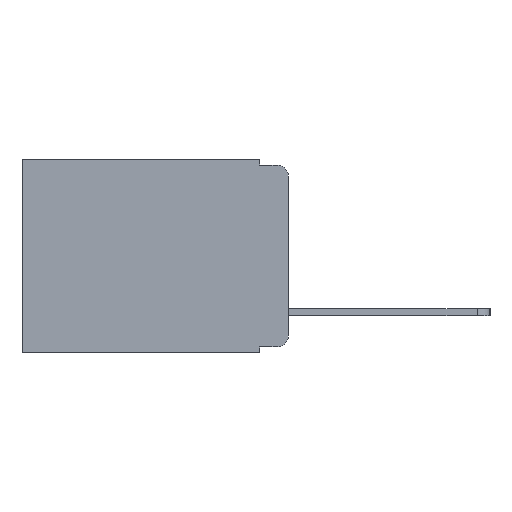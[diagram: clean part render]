
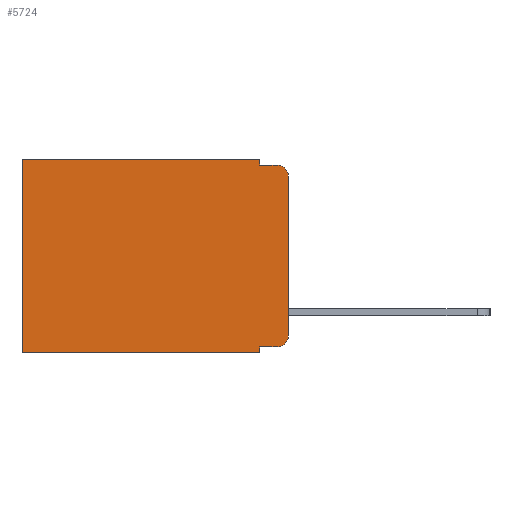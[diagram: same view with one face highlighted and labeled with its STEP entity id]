
A CAD part, left-side view. The second image highlights one B-rep face of the part: STEP entity #5724.
In plain terms, the highlighted planar face has unit normal (-1, 0, 0).
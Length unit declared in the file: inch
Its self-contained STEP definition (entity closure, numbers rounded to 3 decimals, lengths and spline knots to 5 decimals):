
#82 = ORIENTED_EDGE ( 'NONE', *, *, #8377, .T. ) ;
#190 = ORIENTED_EDGE ( 'NONE', *, *, #8359, .F. ) ;
#415 = VERTEX_POINT ( 'NONE', #7577 ) ;
#423 = DIRECTION ( 'NONE',  ( 0., 0., -1. ) ) ;
#771 = VERTEX_POINT ( 'NONE', #3663 ) ;
#979 = ORIENTED_EDGE ( 'NONE', *, *, #1077, .F. ) ;
#1007 = ORIENTED_EDGE ( 'NONE', *, *, #5299, .T. ) ;
#1014 = CARTESIAN_POINT ( 'NONE',  ( 0.298, 0.02, -0.333 ) ) ;
#1077 = EDGE_CURVE ( 'NONE', #7896, #415, #3103, .T. ) ;
#1097 = CARTESIAN_POINT ( 'NONE',  ( 0.298, 0.473, 0. ) ) ;
#1427 = DIRECTION ( 'NONE',  ( 0., 1., 0. ) ) ;
#1825 = DIRECTION ( 'NONE',  ( 0., 0., -1. ) ) ;
#1996 = AXIS2_PLACEMENT_3D ( 'NONE', #7749, #2666, #8629 ) ;
#2127 = VERTEX_POINT ( 'NONE', #1014 ) ;
#2159 = CARTESIAN_POINT ( 'NONE',  ( 0.298, 0.051, -0.01 ) ) ;
#2296 = ORIENTED_EDGE ( 'NONE', *, *, #4402, .T. ) ;
#2313 = DIRECTION ( 'NONE',  ( 0., -1., 0. ) ) ;
#2457 = ORIENTED_EDGE ( 'NONE', *, *, #10166, .T. ) ;
#2502 = VERTEX_POINT ( 'NONE', #7843 ) ;
#2626 = DIRECTION ( 'NONE',  ( 0., 1., 0. ) ) ;
#2666 = DIRECTION ( 'NONE',  ( -1., 0., 0. ) ) ;
#2675 = CARTESIAN_POINT ( 'NONE',  ( 0.298, 0., -0.03 ) ) ;
#2766 = CARTESIAN_POINT ( 'NONE',  ( 0.298, 0.473, 0. ) ) ;
#2996 = LINE ( 'NONE', #6243, #9553 ) ;
#3103 = LINE ( 'NONE', #9639, #4850 ) ;
#3248 = VECTOR ( 'NONE', #6937, 39.37008 ) ;
#3354 = ORIENTED_EDGE ( 'NONE', *, *, #10313, .F. ) ;
#3479 = FACE_OUTER_BOUND ( 'NONE', #9090, .T. ) ;
#3663 = CARTESIAN_POINT ( 'NONE',  ( 0.298, 0.02, -0.01 ) ) ;
#4377 = EDGE_CURVE ( 'NONE', #10200, #8813, #5758, .T. ) ;
#4380 = VERTEX_POINT ( 'NONE', #6906 ) ;
#4402 = EDGE_CURVE ( 'NONE', #2502, #6984, #2996, .T. ) ;
#4721 = CIRCLE ( 'NONE', #7910, 0.02 ) ;
#4850 = VECTOR ( 'NONE', #423, 39.37008 ) ;
#4919 = DIRECTION ( 'NONE',  ( -1., 0., 0. ) ) ;
#5036 = PLANE ( 'NONE',  #10407 ) ;
#5223 = VECTOR ( 'NONE', #8482, 39.37008 ) ;
#5299 = EDGE_CURVE ( 'NONE', #6984, #4380, #9792, .T. ) ;
#5338 = CARTESIAN_POINT ( 'NONE',  ( 0.298, 0.051, 0. ) ) ;
#5356 = LINE ( 'NONE', #6242, #7105 ) ;
#5380 = DIRECTION ( 'NONE',  ( 0., 0., -1. ) ) ;
#5655 = CIRCLE ( 'NONE', #1996, 0.02 ) ;
#5724 = ADVANCED_FACE ( 'NONE', ( #3479 ), #5036, .F. ) ;
#5758 = LINE ( 'NONE', #5338, #3248 ) ;
#6135 = ORIENTED_EDGE ( 'NONE', *, *, #4377, .F. ) ;
#6159 = ORIENTED_EDGE ( 'NONE', *, *, #10584, .T. ) ;
#6242 = CARTESIAN_POINT ( 'NONE',  ( 0.298, 0.051, 0. ) ) ;
#6243 = CARTESIAN_POINT ( 'NONE',  ( 0.298, 0., 0. ) ) ;
#6434 = VECTOR ( 'NONE', #9492, 39.37008 ) ;
#6581 = CARTESIAN_POINT ( 'NONE',  ( 0.298, 0.051, -0.343 ) ) ;
#6906 = CARTESIAN_POINT ( 'NONE',  ( 0.298, 0.473, -0.343 ) ) ;
#6937 = DIRECTION ( 'NONE',  ( 0., 0., -1. ) ) ;
#6984 = VERTEX_POINT ( 'NONE', #2766 ) ;
#7105 = VECTOR ( 'NONE', #5380, 39.37008 ) ;
#7117 = VECTOR ( 'NONE', #2313, 39.37008 ) ;
#7375 = LINE ( 'NONE', #8262, #7117 ) ;
#7577 = CARTESIAN_POINT ( 'NONE',  ( 0.298, 0., -0.313 ) ) ;
#7719 = CARTESIAN_POINT ( 'NONE',  ( 0.298, 0., -0.343 ) ) ;
#7749 = CARTESIAN_POINT ( 'NONE',  ( 0.298, 0.02, -0.03 ) ) ;
#7833 = DIRECTION ( 'NONE',  ( 1., 0., 0. ) ) ;
#7843 = CARTESIAN_POINT ( 'NONE',  ( 0.298, 0.051, 0. ) ) ;
#7896 = VERTEX_POINT ( 'NONE', #2675 ) ;
#7910 = AXIS2_PLACEMENT_3D ( 'NONE', #10032, #4919, #10851 ) ;
#8150 = ORIENTED_EDGE ( 'NONE', *, *, #9909, .F. ) ;
#8207 = VECTOR ( 'NONE', #2626, 39.37008 ) ;
#8262 = CARTESIAN_POINT ( 'NONE',  ( 0.298, 0.051, -0.01 ) ) ;
#8359 = EDGE_CURVE ( 'NONE', #8813, #4380, #10484, .T. ) ;
#8377 = EDGE_CURVE ( 'NONE', #7896, #771, #5655, .T. ) ;
#8482 = DIRECTION ( 'NONE',  ( 0., 0., -1. ) ) ;
#8614 = CARTESIAN_POINT ( 'NONE',  ( 0.298, 0.051, -0.333 ) ) ;
#8629 = DIRECTION ( 'NONE',  ( 0., 0., -1. ) ) ;
#8813 = VERTEX_POINT ( 'NONE', #6581 ) ;
#9090 = EDGE_LOOP ( 'NONE', ( #979, #82, #8150, #3354, #2296, #1007, #190, #6135, #2457, #6159 ) ) ;
#9418 = CARTESIAN_POINT ( 'NONE',  ( 0.298, 0., 0. ) ) ;
#9492 = DIRECTION ( 'NONE',  ( 0., -1., 0. ) ) ;
#9522 = CARTESIAN_POINT ( 'NONE',  ( 0.298, 0.051, -0.333 ) ) ;
#9553 = VECTOR ( 'NONE', #1427, 39.37008 ) ;
#9639 = CARTESIAN_POINT ( 'NONE',  ( 0.298, 0., 0. ) ) ;
#9792 = LINE ( 'NONE', #1097, #5223 ) ;
#9909 = EDGE_CURVE ( 'NONE', #10448, #771, #7375, .T. ) ;
#10032 = CARTESIAN_POINT ( 'NONE',  ( 0.298, 0.02, -0.313 ) ) ;
#10166 = EDGE_CURVE ( 'NONE', #10200, #2127, #10955, .T. ) ;
#10200 = VERTEX_POINT ( 'NONE', #9522 ) ;
#10313 = EDGE_CURVE ( 'NONE', #2502, #10448, #5356, .T. ) ;
#10407 = AXIS2_PLACEMENT_3D ( 'NONE', #9418, #7833, #1825 ) ;
#10448 = VERTEX_POINT ( 'NONE', #2159 ) ;
#10484 = LINE ( 'NONE', #7719, #8207 ) ;
#10584 = EDGE_CURVE ( 'NONE', #2127, #415, #4721, .T. ) ;
#10851 = DIRECTION ( 'NONE',  ( 0., 0., -1. ) ) ;
#10955 = LINE ( 'NONE', #8614, #6434 ) ;
